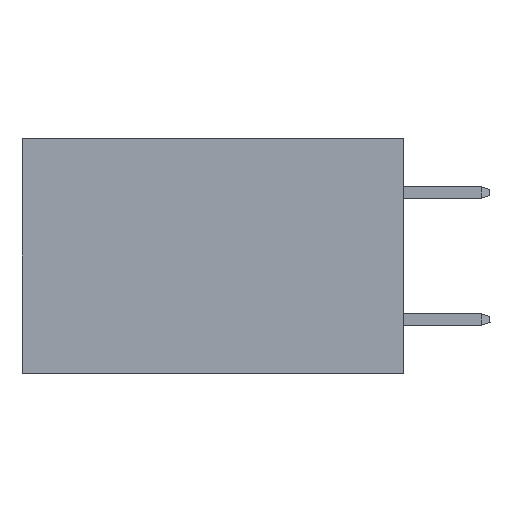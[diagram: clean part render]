
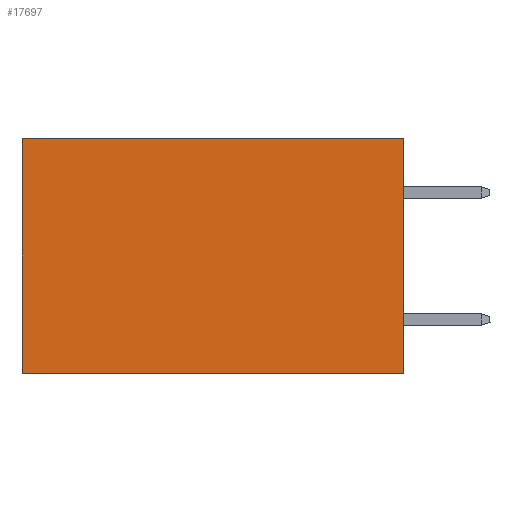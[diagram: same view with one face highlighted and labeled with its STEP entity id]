
A CAD part, left-side view. The second image highlights one B-rep face of the part: STEP entity #17697.
In plain terms, the highlighted planar face has unit normal (-1, 0, 0).
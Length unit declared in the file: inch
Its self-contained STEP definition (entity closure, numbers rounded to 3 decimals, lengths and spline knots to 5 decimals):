
#19 = FACE_OUTER_BOUND ( 'NONE', #22906, .T. ) ;
#1032 = AXIS2_PLACEMENT_3D ( 'NONE', #10581, #5290, #21509 ) ;
#3848 = CARTESIAN_POINT ( 'NONE',  ( 0.2875, 0.6, 0. ) ) ;
#5109 = DIRECTION ( 'NONE',  ( 0., 1., 0. ) ) ;
#5290 = DIRECTION ( 'NONE',  ( 1., 0., 0. ) ) ;
#5424 = VERTEX_POINT ( 'NONE', #18457 ) ;
#5694 = VECTOR ( 'NONE', #20414, 39.37008 ) ;
#5870 = VERTEX_POINT ( 'NONE', #6079 ) ;
#6079 = CARTESIAN_POINT ( 'NONE',  ( 0.2875, 0., 0. ) ) ;
#7009 = DIRECTION ( 'NONE',  ( 0., 0., -1. ) ) ;
#10078 = CARTESIAN_POINT ( 'NONE',  ( 0.2875, 0., 0. ) ) ;
#10423 = VECTOR ( 'NONE', #7009, 39.37008 ) ;
#10466 = ORIENTED_EDGE ( 'NONE', *, *, #14286, .T. ) ;
#10581 = CARTESIAN_POINT ( 'NONE',  ( 0.2875, 0., 0. ) ) ;
#11627 = EDGE_CURVE ( 'NONE', #5870, #5424, #14564, .T. ) ;
#11741 = LINE ( 'NONE', #10078, #12577 ) ;
#11826 = ORIENTED_EDGE ( 'NONE', *, *, #11627, .F. ) ;
#12410 = CARTESIAN_POINT ( 'NONE',  ( 0.2875, 0., 0. ) ) ;
#12577 = VECTOR ( 'NONE', #22990, 39.37008 ) ;
#13445 = CARTESIAN_POINT ( 'NONE',  ( 0.2875, 0.6, 0. ) ) ;
#14252 = LINE ( 'NONE', #21561, #15075 ) ;
#14286 = EDGE_CURVE ( 'NONE', #20723, #23608, #21736, .T. ) ;
#14564 = LINE ( 'NONE', #12410, #10423 ) ;
#15075 = VECTOR ( 'NONE', #5109, 39.37008 ) ;
#15374 = ORIENTED_EDGE ( 'NONE', *, *, #16703, .F. ) ;
#16703 = EDGE_CURVE ( 'NONE', #5424, #23608, #14252, .T. ) ;
#17697 = ADVANCED_FACE ( 'NONE', ( #19 ), #17883, .F. ) ;
#17883 = PLANE ( 'NONE',  #1032 ) ;
#18371 = CARTESIAN_POINT ( 'NONE',  ( 0.2875, 0.6, -0.37 ) ) ;
#18433 = EDGE_CURVE ( 'NONE', #5870, #20723, #11741, .T. ) ;
#18457 = CARTESIAN_POINT ( 'NONE',  ( 0.2875, 0., -0.37 ) ) ;
#18999 = ORIENTED_EDGE ( 'NONE', *, *, #18433, .T. ) ;
#20414 = DIRECTION ( 'NONE',  ( 0., 0., -1. ) ) ;
#20723 = VERTEX_POINT ( 'NONE', #13445 ) ;
#21509 = DIRECTION ( 'NONE',  ( 0., 0., -1. ) ) ;
#21561 = CARTESIAN_POINT ( 'NONE',  ( 0.2875, 0., -0.37 ) ) ;
#21736 = LINE ( 'NONE', #3848, #5694 ) ;
#22906 = EDGE_LOOP ( 'NONE', ( #10466, #15374, #11826, #18999 ) ) ;
#22990 = DIRECTION ( 'NONE',  ( 0., 1., 0. ) ) ;
#23608 = VERTEX_POINT ( 'NONE', #18371 ) ;
